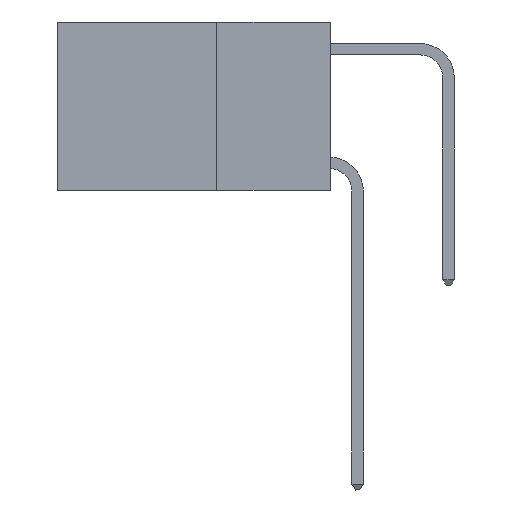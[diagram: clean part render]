
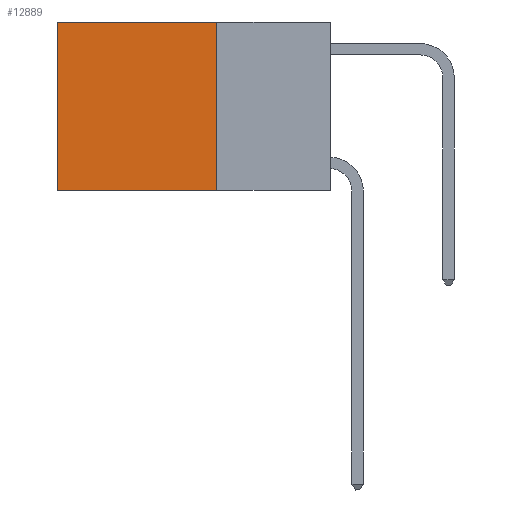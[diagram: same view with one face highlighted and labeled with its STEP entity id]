
A CAD part, left-side view. The second image highlights one B-rep face of the part: STEP entity #12889.
In plain terms, the highlighted planar face has unit normal (-1, 0, 0).
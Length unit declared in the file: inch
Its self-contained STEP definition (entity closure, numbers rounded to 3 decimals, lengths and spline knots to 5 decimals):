
#926 = ORIENTED_EDGE ( 'NONE', *, *, #14862, .T. ) ;
#1043 = CARTESIAN_POINT ( 'NONE',  ( 0.2625, 0.6, 0. ) ) ;
#1561 = ORIENTED_EDGE ( 'NONE', *, *, #11378, .F. ) ;
#2248 = CARTESIAN_POINT ( 'NONE',  ( 0.2625, 0.25, 0. ) ) ;
#2851 = CARTESIAN_POINT ( 'NONE',  ( 0.2625, 0.25, 0. ) ) ;
#2942 = VECTOR ( 'NONE', #10928, 39.37008 ) ;
#3692 = LINE ( 'NONE', #9737, #2942 ) ;
#4257 = VECTOR ( 'NONE', #6548, 39.37008 ) ;
#4769 = VERTEX_POINT ( 'NONE', #13016 ) ;
#4995 = ORIENTED_EDGE ( 'NONE', *, *, #6237, .F. ) ;
#5004 = VERTEX_POINT ( 'NONE', #2851 ) ;
#5299 = EDGE_CURVE ( 'NONE', #5004, #11762, #11721, .T. ) ;
#5519 = VECTOR ( 'NONE', #8106, 39.37008 ) ;
#6237 = EDGE_CURVE ( 'NONE', #6272, #4769, #11330, .T. ) ;
#6272 = VERTEX_POINT ( 'NONE', #14349 ) ;
#6548 = DIRECTION ( 'NONE',  ( 0., 0., -1. ) ) ;
#6634 = DIRECTION ( 'NONE',  ( 1., 0., 0. ) ) ;
#8106 = DIRECTION ( 'NONE',  ( 0., 1., 0. ) ) ;
#9670 = FACE_OUTER_BOUND ( 'NONE', #11817, .T. ) ;
#9737 = CARTESIAN_POINT ( 'NONE',  ( 0.2625, 0.25, 0. ) ) ;
#9966 = CARTESIAN_POINT ( 'NONE',  ( 0.2625, 0.6, 0. ) ) ;
#10054 = PLANE ( 'NONE',  #12878 ) ;
#10867 = DIRECTION ( 'NONE',  ( 0., 1., 0. ) ) ;
#10928 = DIRECTION ( 'NONE',  ( 0., 0., -1. ) ) ;
#11330 = LINE ( 'NONE', #13176, #14022 ) ;
#11378 = EDGE_CURVE ( 'NONE', #5004, #6272, #3692, .T. ) ;
#11721 = LINE ( 'NONE', #2248, #5519 ) ;
#11762 = VERTEX_POINT ( 'NONE', #1043 ) ;
#11817 = EDGE_LOOP ( 'NONE', ( #926, #4995, #1561, #15177 ) ) ;
#12878 = AXIS2_PLACEMENT_3D ( 'NONE', #13578, #6634, #14717 ) ;
#12889 = ADVANCED_FACE ( 'NONE', ( #9670 ), #10054, .F. ) ;
#13016 = CARTESIAN_POINT ( 'NONE',  ( 0.2625, 0.6, -0.37 ) ) ;
#13176 = CARTESIAN_POINT ( 'NONE',  ( 0.2625, 0.25, -0.37 ) ) ;
#13578 = CARTESIAN_POINT ( 'NONE',  ( 0.2625, 0.25, 0. ) ) ;
#13917 = LINE ( 'NONE', #9966, #4257 ) ;
#14022 = VECTOR ( 'NONE', #10867, 39.37008 ) ;
#14349 = CARTESIAN_POINT ( 'NONE',  ( 0.2625, 0.25, -0.37 ) ) ;
#14717 = DIRECTION ( 'NONE',  ( 0., 0., -1. ) ) ;
#14862 = EDGE_CURVE ( 'NONE', #11762, #4769, #13917, .T. ) ;
#15177 = ORIENTED_EDGE ( 'NONE', *, *, #5299, .T. ) ;
